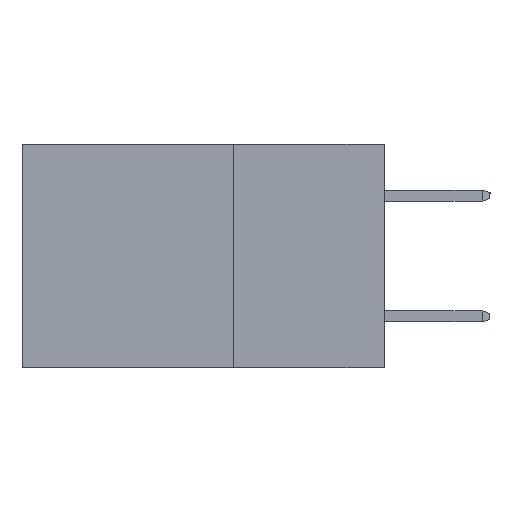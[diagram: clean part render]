
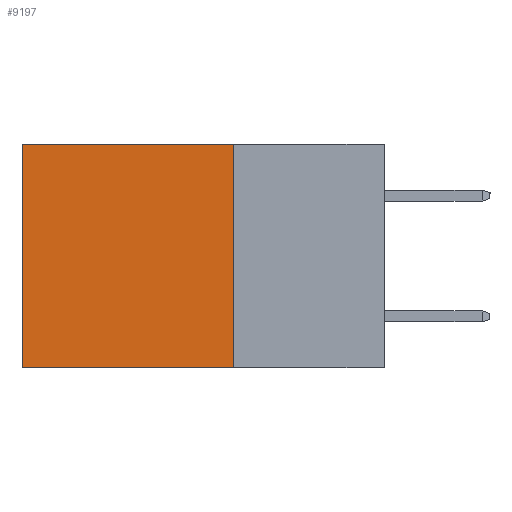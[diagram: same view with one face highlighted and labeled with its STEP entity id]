
A CAD part, left-side view. The second image highlights one B-rep face of the part: STEP entity #9197.
In plain terms, the highlighted planar face has unit normal (-1, 0, 0).
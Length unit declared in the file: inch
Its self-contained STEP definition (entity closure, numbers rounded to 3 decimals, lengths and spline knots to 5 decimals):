
#1114 = CARTESIAN_POINT ( 'NONE',  ( 0.2615, 0.6, 0. ) ) ;
#1345 = EDGE_CURVE ( 'NONE', #7442, #6361, #3594, .T. ) ;
#2809 = VECTOR ( 'NONE', #10776, 39.37008 ) ;
#3315 = CARTESIAN_POINT ( 'NONE',  ( 0.2615, 0.25, -0.37 ) ) ;
#3361 = DIRECTION ( 'NONE',  ( 0., 0., -1. ) ) ;
#3594 = LINE ( 'NONE', #19325, #14758 ) ;
#4231 = FACE_OUTER_BOUND ( 'NONE', #10279, .T. ) ;
#4341 = CARTESIAN_POINT ( 'NONE',  ( 0.2615, 0.25, -0.37 ) ) ;
#4393 = VECTOR ( 'NONE', #4510, 39.37008 ) ;
#4510 = DIRECTION ( 'NONE',  ( 0., 1., 0. ) ) ;
#4821 = LINE ( 'NONE', #3315, #6199 ) ;
#4961 = CARTESIAN_POINT ( 'NONE',  ( 0.2615, 0.25, 0. ) ) ;
#5298 = CARTESIAN_POINT ( 'NONE',  ( 0.2615, 0.25, -0.37 ) ) ;
#6199 = VECTOR ( 'NONE', #12289, 39.37008 ) ;
#6361 = VERTEX_POINT ( 'NONE', #22836 ) ;
#7247 = EDGE_CURVE ( 'NONE', #11381, #12219, #19651, .T. ) ;
#7442 = VERTEX_POINT ( 'NONE', #1114 ) ;
#8898 = ORIENTED_EDGE ( 'NONE', *, *, #13785, .T. ) ;
#9197 = ADVANCED_FACE ( 'NONE', ( #4231 ), #19975, .F. ) ;
#10253 = EDGE_CURVE ( 'NONE', #12219, #6361, #4821, .T. ) ;
#10279 = EDGE_LOOP ( 'NONE', ( #16624, #12473, #10480, #8898 ) ) ;
#10480 = ORIENTED_EDGE ( 'NONE', *, *, #7247, .F. ) ;
#10776 = DIRECTION ( 'NONE',  ( 0., 0., -1. ) ) ;
#10940 = CARTESIAN_POINT ( 'NONE',  ( 0.2615, 0.25, -0.37 ) ) ;
#11343 = DIRECTION ( 'NONE',  ( 0., 0., -1. ) ) ;
#11381 = VERTEX_POINT ( 'NONE', #4961 ) ;
#12219 = VERTEX_POINT ( 'NONE', #10940 ) ;
#12289 = DIRECTION ( 'NONE',  ( 0., 1., 0. ) ) ;
#12473 = ORIENTED_EDGE ( 'NONE', *, *, #10253, .F. ) ;
#13392 = LINE ( 'NONE', #22481, #4393 ) ;
#13785 = EDGE_CURVE ( 'NONE', #11381, #7442, #13392, .T. ) ;
#14758 = VECTOR ( 'NONE', #3361, 39.37008 ) ;
#15082 = DIRECTION ( 'NONE',  ( 1., 0., 0. ) ) ;
#16624 = ORIENTED_EDGE ( 'NONE', *, *, #1345, .T. ) ;
#19325 = CARTESIAN_POINT ( 'NONE',  ( 0.2615, 0.6, -0.37 ) ) ;
#19651 = LINE ( 'NONE', #5298, #2809 ) ;
#19975 = PLANE ( 'NONE',  #22964 ) ;
#22481 = CARTESIAN_POINT ( 'NONE',  ( 0.2615, 0.25, 0. ) ) ;
#22836 = CARTESIAN_POINT ( 'NONE',  ( 0.2615, 0.6, -0.37 ) ) ;
#22964 = AXIS2_PLACEMENT_3D ( 'NONE', #4341, #15082, #11343 ) ;
